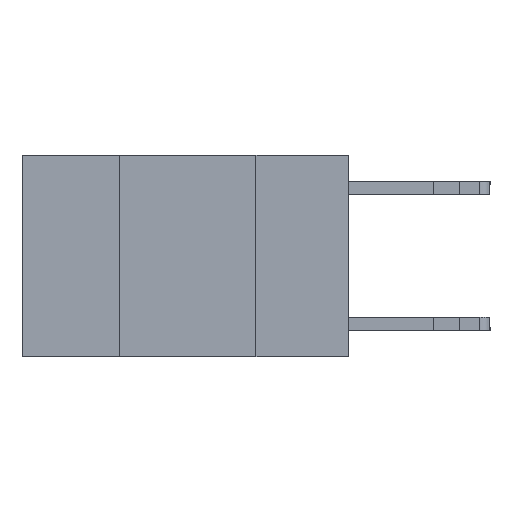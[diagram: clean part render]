
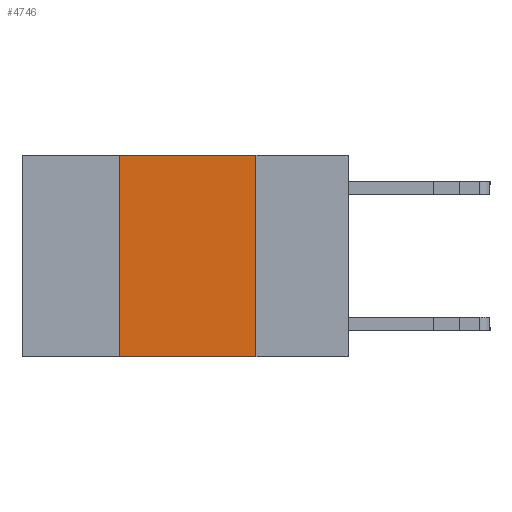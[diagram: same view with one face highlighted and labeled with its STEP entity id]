
A CAD part, left-side view. The second image highlights one B-rep face of the part: STEP entity #4746.
In plain terms, the highlighted planar face has unit normal (-1, 0, 0).
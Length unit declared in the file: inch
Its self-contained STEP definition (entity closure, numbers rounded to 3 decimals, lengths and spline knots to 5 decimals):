
#785 = CARTESIAN_POINT ( 'NONE',  ( 0., 0.6, 0. ) ) ;
#1614 = LINE ( 'NONE', #17188, #18393 ) ;
#2312 = VECTOR ( 'NONE', #13946, 39.37008 ) ;
#2998 = EDGE_CURVE ( 'NONE', #9956, #20788, #24275, .T. ) ;
#3181 = ORIENTED_EDGE ( 'NONE', *, *, #2998, .F. ) ;
#3606 = ORIENTED_EDGE ( 'NONE', *, *, #11807, .F. ) ;
#3738 = CARTESIAN_POINT ( 'NONE',  ( 0., 0.42, -0.37 ) ) ;
#3892 = DIRECTION ( 'NONE',  ( 0., 0., 1. ) ) ;
#4142 = DIRECTION ( 'NONE',  ( 0., 0., -1. ) ) ;
#4288 = FACE_OUTER_BOUND ( 'NONE', #21532, .T. ) ;
#4746 = ADVANCED_FACE ( 'NONE', ( #4288 ), #24105, .F. ) ;
#5348 = EDGE_CURVE ( 'NONE', #14528, #21109, #11881, .T. ) ;
#6127 = CARTESIAN_POINT ( 'NONE',  ( 0., 0.42, 0. ) ) ;
#8547 = DIRECTION ( 'NONE',  ( 0., 0., -1. ) ) ;
#9584 = AXIS2_PLACEMENT_3D ( 'NONE', #15621, #17470, #8547 ) ;
#9956 = VERTEX_POINT ( 'NONE', #6127 ) ;
#10418 = LINE ( 'NONE', #14668, #18366 ) ;
#11320 = EDGE_CURVE ( 'NONE', #14528, #9956, #10418, .T. ) ;
#11807 = EDGE_CURVE ( 'NONE', #20788, #21109, #1614, .T. ) ;
#11881 = LINE ( 'NONE', #24773, #18198 ) ;
#12172 = CARTESIAN_POINT ( 'NONE',  ( 0., 0.17, -0.37 ) ) ;
#13880 = DIRECTION ( 'NONE',  ( 0., -1., 0. ) ) ;
#13946 = DIRECTION ( 'NONE',  ( 0., -1., 0. ) ) ;
#14528 = VERTEX_POINT ( 'NONE', #3738 ) ;
#14668 = CARTESIAN_POINT ( 'NONE',  ( 0., 0.42, 0. ) ) ;
#15621 = CARTESIAN_POINT ( 'NONE',  ( 0., 0.6, 0. ) ) ;
#17188 = CARTESIAN_POINT ( 'NONE',  ( 0., 0.17, 0. ) ) ;
#17470 = DIRECTION ( 'NONE',  ( 1., 0., 0. ) ) ;
#17650 = ORIENTED_EDGE ( 'NONE', *, *, #11320, .F. ) ;
#18198 = VECTOR ( 'NONE', #13880, 39.37008 ) ;
#18366 = VECTOR ( 'NONE', #3892, 39.37008 ) ;
#18393 = VECTOR ( 'NONE', #4142, 39.37008 ) ;
#20788 = VERTEX_POINT ( 'NONE', #21973 ) ;
#21109 = VERTEX_POINT ( 'NONE', #12172 ) ;
#21532 = EDGE_LOOP ( 'NONE', ( #3606, #3181, #17650, #23155 ) ) ;
#21973 = CARTESIAN_POINT ( 'NONE',  ( 0., 0.17, 0. ) ) ;
#23155 = ORIENTED_EDGE ( 'NONE', *, *, #5348, .T. ) ;
#24105 = PLANE ( 'NONE',  #9584 ) ;
#24275 = LINE ( 'NONE', #785, #2312 ) ;
#24773 = CARTESIAN_POINT ( 'NONE',  ( 0., 0.6, -0.37 ) ) ;
